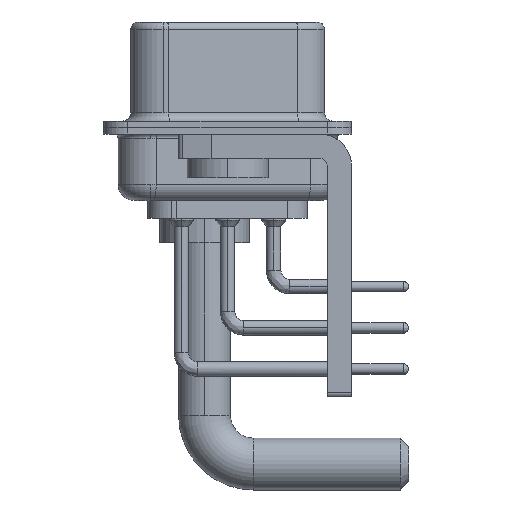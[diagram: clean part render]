
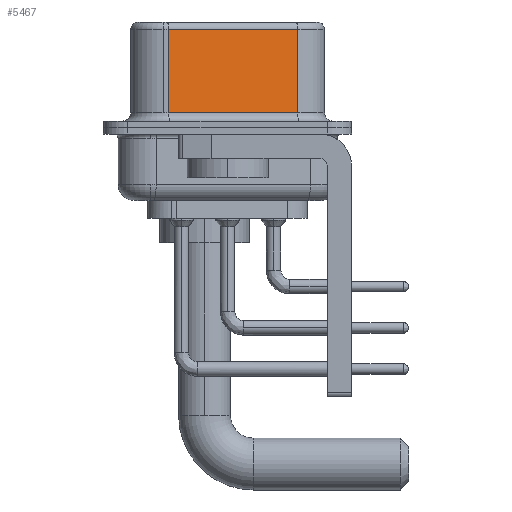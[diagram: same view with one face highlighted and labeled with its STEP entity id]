
A CAD part, left-side view. The second image highlights one B-rep face of the part: STEP entity #5467.
In plain terms, the highlighted planar face has unit normal (-0.985, -0.174, 0).
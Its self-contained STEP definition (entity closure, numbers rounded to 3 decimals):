
#434 = DIRECTION ( 'NONE',  ( -0.174, 0.985, 0. ) ) ;
#1932 = VERTEX_POINT ( 'NONE', #36374 ) ;
#2264 = VERTEX_POINT ( 'NONE', #7817 ) ;
#5467 = ADVANCED_FACE ( 'NONE', ( #35785 ), #35976, .F. ) ;
#5740 = DIRECTION ( 'NONE',  ( 0., 0., -1. ) ) ;
#6808 = VECTOR ( 'NONE', #10009, 1000. ) ;
#7180 = VECTOR ( 'NONE', #5740, 1000. ) ;
#7817 = CARTESIAN_POINT ( 'NONE',  ( 3.73, 3.628, 0.9 ) ) ;
#7950 = EDGE_CURVE ( 'NONE', #1932, #23365, #22609, .T. ) ;
#9408 = DIRECTION ( 'NONE',  ( -0.174, 0.985, 0. ) ) ;
#9915 = LINE ( 'NONE', #18456, #19219 ) ;
#9985 = CARTESIAN_POINT ( 'NONE',  ( 5.132, -4.322, 0.9 ) ) ;
#10009 = DIRECTION ( 'NONE',  ( 0., 0., -1. ) ) ;
#10662 = EDGE_CURVE ( 'NONE', #2264, #23365, #25471, .T. ) ;
#12096 = ORIENTED_EDGE ( 'NONE', *, *, #29636, .T. ) ;
#13838 = ORIENTED_EDGE ( 'NONE', *, *, #29384, .T. ) ;
#17294 = CARTESIAN_POINT ( 'NONE',  ( 5.132, -4.322, 0.9 ) ) ;
#18456 = CARTESIAN_POINT ( 'NONE',  ( 5.132, -4.322, 6.02 ) ) ;
#19219 = VECTOR ( 'NONE', #434, 1000. ) ;
#20124 = AXIS2_PLACEMENT_3D ( 'NONE', #26308, #32688, #9408 ) ;
#20261 = VECTOR ( 'NONE', #30729, 1000. ) ;
#22609 = LINE ( 'NONE', #38145, #7180 ) ;
#23365 = VERTEX_POINT ( 'NONE', #17294 ) ;
#25471 = LINE ( 'NONE', #9985, #20261 ) ;
#25854 = LINE ( 'NONE', #27660, #6808 ) ;
#26308 = CARTESIAN_POINT ( 'NONE',  ( 5.132, -4.322, 6.52 ) ) ;
#26518 = EDGE_LOOP ( 'NONE', ( #37906, #12096, #13838, #35566 ) ) ;
#27660 = CARTESIAN_POINT ( 'NONE',  ( 3.73, 3.628, 6.52 ) ) ;
#29384 = EDGE_CURVE ( 'NONE', #31510, #2264, #25854, .T. ) ;
#29636 = EDGE_CURVE ( 'NONE', #1932, #31510, #9915, .T. ) ;
#30729 = DIRECTION ( 'NONE',  ( 0.174, -0.985, 0. ) ) ;
#31510 = VERTEX_POINT ( 'NONE', #37294 ) ;
#32688 = DIRECTION ( 'NONE',  ( 0.985, 0.174, 0. ) ) ;
#35566 = ORIENTED_EDGE ( 'NONE', *, *, #10662, .T. ) ;
#35785 = FACE_OUTER_BOUND ( 'NONE', #26518, .T. ) ;
#35976 = PLANE ( 'NONE',  #20124 ) ;
#36374 = CARTESIAN_POINT ( 'NONE',  ( 5.132, -4.322, 6.02 ) ) ;
#37294 = CARTESIAN_POINT ( 'NONE',  ( 3.73, 3.628, 6.02 ) ) ;
#37906 = ORIENTED_EDGE ( 'NONE', *, *, #7950, .F. ) ;
#38145 = CARTESIAN_POINT ( 'NONE',  ( 5.132, -4.322, 6.52 ) ) ;
